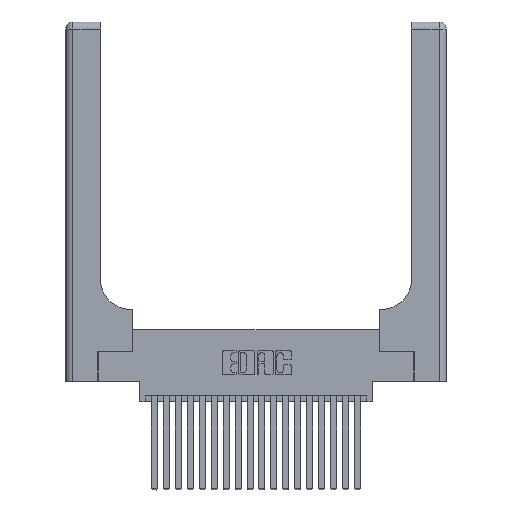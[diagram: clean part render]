
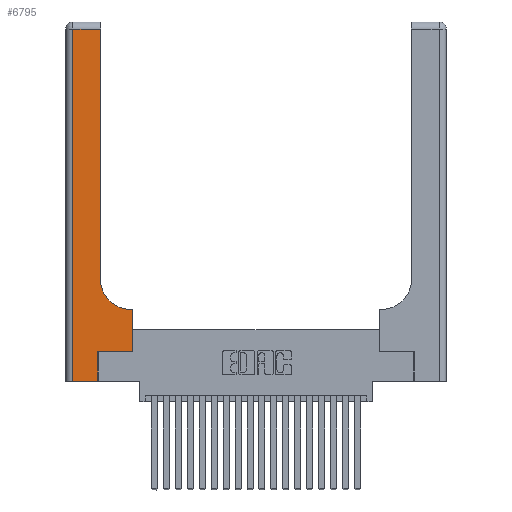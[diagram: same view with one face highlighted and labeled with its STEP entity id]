
A CAD part, top view. The second image highlights one B-rep face of the part: STEP entity #6795.
In plain terms, the highlighted planar face has unit normal (0, 0, 1).
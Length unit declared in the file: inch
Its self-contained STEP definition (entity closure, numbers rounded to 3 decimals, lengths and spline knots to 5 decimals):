
#10 = VERTEX_POINT ( 'NONE', #1258 ) ;
#877 = CARTESIAN_POINT ( 'NONE',  ( 0.2915, 0.6, 0.37 ) ) ;
#956 = DIRECTION ( 'NONE',  ( 0., 1., 0. ) ) ;
#1258 = CARTESIAN_POINT ( 'NONE',  ( 0.269, 0.25, 0.37 ) ) ;
#1290 = VERTEX_POINT ( 'NONE', #6863 ) ;
#1336 = DIRECTION ( 'NONE',  ( 1., 0., 0. ) ) ;
#1384 = LINE ( 'NONE', #6046, #17143 ) ;
#1605 = EDGE_CURVE ( 'NONE', #15163, #21498, #16390, .T. ) ;
#1759 = ORIENTED_EDGE ( 'NONE', *, *, #6299, .T. ) ;
#2442 = EDGE_CURVE ( 'NONE', #9604, #10, #16634, .T. ) ;
#2456 = DIRECTION ( 'NONE',  ( -1., 0., 0. ) ) ;
#2644 = DIRECTION ( 'NONE',  ( 0., -1., 0. ) ) ;
#3459 = DIRECTION ( 'NONE',  ( 0., 0., -1. ) ) ;
#3637 = VERTEX_POINT ( 'NONE', #9667 ) ;
#3734 = ORIENTED_EDGE ( 'NONE', *, *, #7463, .T. ) ;
#3769 = LINE ( 'NONE', #19675, #18728 ) ;
#4354 = DIRECTION ( 'NONE',  ( 0., 1., 0. ) ) ;
#4548 = EDGE_LOOP ( 'NONE', ( #15620, #5377, #3734, #1759, #18813, #13268, #16971, #17579, #13659 ) ) ;
#5377 = ORIENTED_EDGE ( 'NONE', *, *, #18556, .T. ) ;
#6046 = CARTESIAN_POINT ( 'NONE',  ( 0., 2.94, 0.37 ) ) ;
#6149 = LINE ( 'NONE', #11773, #11321 ) ;
#6299 = EDGE_CURVE ( 'NONE', #21782, #9604, #6149, .T. ) ;
#6515 = DIRECTION ( 'NONE',  ( -1., 0., 0. ) ) ;
#6692 = EDGE_CURVE ( 'NONE', #10, #1290, #19399, .T. ) ;
#6795 = ADVANCED_FACE ( 'NONE', ( #16133 ), #7739, .F. ) ;
#6863 = CARTESIAN_POINT ( 'NONE',  ( 0.5585, 0.25, 0.37 ) ) ;
#7410 = VERTEX_POINT ( 'NONE', #11190 ) ;
#7463 = EDGE_CURVE ( 'NONE', #7410, #21782, #11807, .T. ) ;
#7739 = PLANE ( 'NONE',  #13614 ) ;
#8212 = LINE ( 'NONE', #877, #11996 ) ;
#8340 = VECTOR ( 'NONE', #12576, 39.37008 ) ;
#9244 = CARTESIAN_POINT ( 'NONE',  ( 0., 3., 0.37 ) ) ;
#9569 = EDGE_CURVE ( 'NONE', #1290, #14589, #20119, .T. ) ;
#9604 = VERTEX_POINT ( 'NONE', #20001 ) ;
#9667 = CARTESIAN_POINT ( 'NONE',  ( 0.2915, 2.94, 0.37 ) ) ;
#9699 = EDGE_CURVE ( 'NONE', #14589, #15163, #8212, .T. ) ;
#10844 = DIRECTION ( 'NONE',  ( -1., 0., 0. ) ) ;
#11190 = CARTESIAN_POINT ( 'NONE',  ( 0.06, 2.94, 0.37 ) ) ;
#11321 = VECTOR ( 'NONE', #1336, 39.37008 ) ;
#11381 = CARTESIAN_POINT ( 'NONE',  ( 0.5585, 0.25, 0.37 ) ) ;
#11773 = CARTESIAN_POINT ( 'NONE',  ( 0., 0., 0.37 ) ) ;
#11807 = LINE ( 'NONE', #21889, #14207 ) ;
#11996 = VECTOR ( 'NONE', #6515, 39.37008 ) ;
#12040 = VECTOR ( 'NONE', #4354, 39.37008 ) ;
#12576 = DIRECTION ( 'NONE',  ( 1., 0., 0. ) ) ;
#13268 = ORIENTED_EDGE ( 'NONE', *, *, #6692, .T. ) ;
#13271 = EDGE_CURVE ( 'NONE', #21498, #3637, #3769, .T. ) ;
#13560 = CARTESIAN_POINT ( 'NONE',  ( 0.2915, 0.85, 0.37 ) ) ;
#13614 = AXIS2_PLACEMENT_3D ( 'NONE', #9244, #19846, #10844 ) ;
#13659 = ORIENTED_EDGE ( 'NONE', *, *, #1605, .T. ) ;
#13954 = AXIS2_PLACEMENT_3D ( 'NONE', #20636, #3459, #17428 ) ;
#14207 = VECTOR ( 'NONE', #2644, 39.37008 ) ;
#14589 = VERTEX_POINT ( 'NONE', #18643 ) ;
#14739 = CARTESIAN_POINT ( 'NONE',  ( 0.269, 0., 0.37 ) ) ;
#15163 = VERTEX_POINT ( 'NONE', #16868 ) ;
#15620 = ORIENTED_EDGE ( 'NONE', *, *, #13271, .T. ) ;
#16133 = FACE_OUTER_BOUND ( 'NONE', #4548, .T. ) ;
#16329 = CARTESIAN_POINT ( 'NONE',  ( 0.269, 0.25, 0.37 ) ) ;
#16390 = CIRCLE ( 'NONE', #13954, 0.25 ) ;
#16634 = LINE ( 'NONE', #14739, #12040 ) ;
#16868 = CARTESIAN_POINT ( 'NONE',  ( 0.5415, 0.6, 0.37 ) ) ;
#16971 = ORIENTED_EDGE ( 'NONE', *, *, #9569, .T. ) ;
#17143 = VECTOR ( 'NONE', #2456, 39.37008 ) ;
#17428 = DIRECTION ( 'NONE',  ( 1., 0., 0. ) ) ;
#17579 = ORIENTED_EDGE ( 'NONE', *, *, #9699, .T. ) ;
#17931 = VECTOR ( 'NONE', #956, 39.37008 ) ;
#18002 = CARTESIAN_POINT ( 'NONE',  ( 0.06, 0., 0.37 ) ) ;
#18556 = EDGE_CURVE ( 'NONE', #3637, #7410, #1384, .T. ) ;
#18643 = CARTESIAN_POINT ( 'NONE',  ( 0.5585, 0.6, 0.37 ) ) ;
#18728 = VECTOR ( 'NONE', #19518, 39.37008 ) ;
#18813 = ORIENTED_EDGE ( 'NONE', *, *, #2442, .T. ) ;
#19399 = LINE ( 'NONE', #16329, #8340 ) ;
#19518 = DIRECTION ( 'NONE',  ( 0., 1., 0. ) ) ;
#19675 = CARTESIAN_POINT ( 'NONE',  ( 0.2915, 3., 0.37 ) ) ;
#19846 = DIRECTION ( 'NONE',  ( 0., 0., -1. ) ) ;
#20001 = CARTESIAN_POINT ( 'NONE',  ( 0.269, 0., 0.37 ) ) ;
#20119 = LINE ( 'NONE', #11381, #17931 ) ;
#20636 = CARTESIAN_POINT ( 'NONE',  ( 0.5415, 0.85, 0.37 ) ) ;
#21498 = VERTEX_POINT ( 'NONE', #13560 ) ;
#21782 = VERTEX_POINT ( 'NONE', #18002 ) ;
#21889 = CARTESIAN_POINT ( 'NONE',  ( 0.06, 3., 0.37 ) ) ;
